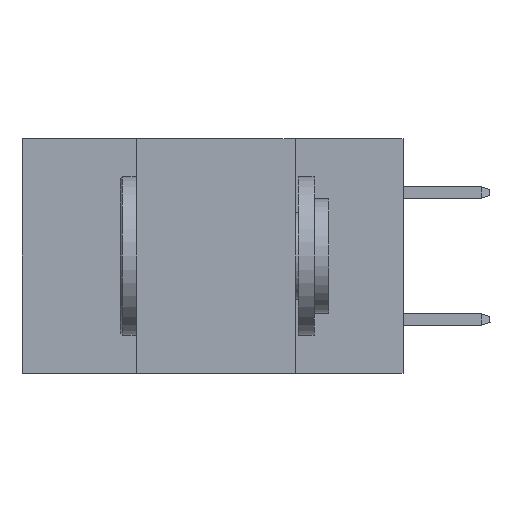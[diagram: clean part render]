
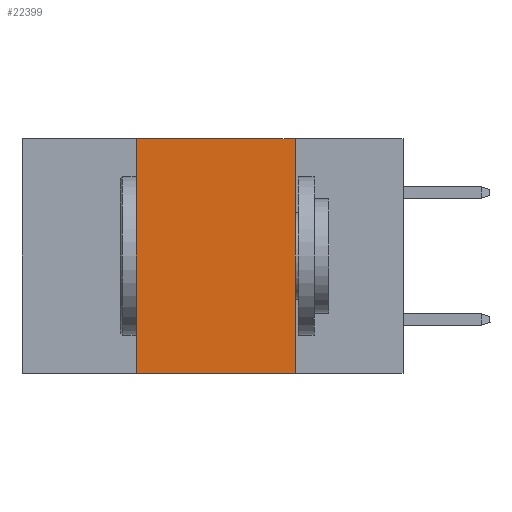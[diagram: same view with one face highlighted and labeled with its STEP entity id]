
A CAD part, left-side view. The second image highlights one B-rep face of the part: STEP entity #22399.
In plain terms, the highlighted planar face has unit normal (-1, 0, 0).
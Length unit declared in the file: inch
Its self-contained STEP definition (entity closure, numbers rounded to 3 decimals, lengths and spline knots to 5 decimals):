
#373 = CARTESIAN_POINT ( 'NONE',  ( 0., 0.17, -0.37 ) ) ;
#2007 = CARTESIAN_POINT ( 'NONE',  ( 0., 0.42, 0. ) ) ;
#2134 = VERTEX_POINT ( 'NONE', #7470 ) ;
#2902 = DIRECTION ( 'NONE',  ( 0., 0., -1. ) ) ;
#3589 = LINE ( 'NONE', #2007, #17598 ) ;
#4139 = VECTOR ( 'NONE', #4787, 39.37008 ) ;
#4154 = VERTEX_POINT ( 'NONE', #8705 ) ;
#4673 = AXIS2_PLACEMENT_3D ( 'NONE', #7321, #22321, #2902 ) ;
#4787 = DIRECTION ( 'NONE',  ( 0., -1., 0. ) ) ;
#5697 = LINE ( 'NONE', #11963, #20404 ) ;
#7186 = PLANE ( 'NONE',  #4673 ) ;
#7321 = CARTESIAN_POINT ( 'NONE',  ( 0., 0.6, 0. ) ) ;
#7470 = CARTESIAN_POINT ( 'NONE',  ( 0., 0.42, 0. ) ) ;
#8705 = CARTESIAN_POINT ( 'NONE',  ( 0., 0.42, -0.37 ) ) ;
#9204 = ORIENTED_EDGE ( 'NONE', *, *, #15856, .F. ) ;
#9379 = VERTEX_POINT ( 'NONE', #373 ) ;
#10395 = VECTOR ( 'NONE', #20916, 39.37008 ) ;
#11452 = EDGE_CURVE ( 'NONE', #4154, #2134, #3589, .T. ) ;
#11963 = CARTESIAN_POINT ( 'NONE',  ( 0., 0.6, -0.37 ) ) ;
#13821 = EDGE_CURVE ( 'NONE', #2134, #18357, #23909, .T. ) ;
#15856 = EDGE_CURVE ( 'NONE', #18357, #9379, #24120, .T. ) ;
#17598 = VECTOR ( 'NONE', #21293, 39.37008 ) ;
#18129 = ORIENTED_EDGE ( 'NONE', *, *, #11452, .F. ) ;
#18357 = VERTEX_POINT ( 'NONE', #27439 ) ;
#19075 = CARTESIAN_POINT ( 'NONE',  ( 0., 0.17, 0. ) ) ;
#19804 = CARTESIAN_POINT ( 'NONE',  ( 0., 0.6, 0. ) ) ;
#19827 = EDGE_CURVE ( 'NONE', #4154, #9379, #5697, .T. ) ;
#20404 = VECTOR ( 'NONE', #25233, 39.37008 ) ;
#20850 = EDGE_LOOP ( 'NONE', ( #9204, #24859, #18129, #23736 ) ) ;
#20916 = DIRECTION ( 'NONE',  ( 0., 0., -1. ) ) ;
#21293 = DIRECTION ( 'NONE',  ( 0., 0., 1. ) ) ;
#22321 = DIRECTION ( 'NONE',  ( 1., 0., 0. ) ) ;
#22399 = ADVANCED_FACE ( 'NONE', ( #26562 ), #7186, .F. ) ;
#23736 = ORIENTED_EDGE ( 'NONE', *, *, #19827, .T. ) ;
#23909 = LINE ( 'NONE', #19804, #4139 ) ;
#24120 = LINE ( 'NONE', #19075, #10395 ) ;
#24859 = ORIENTED_EDGE ( 'NONE', *, *, #13821, .F. ) ;
#25233 = DIRECTION ( 'NONE',  ( 0., -1., 0. ) ) ;
#26562 = FACE_OUTER_BOUND ( 'NONE', #20850, .T. ) ;
#27439 = CARTESIAN_POINT ( 'NONE',  ( 0., 0.17, 0. ) ) ;
